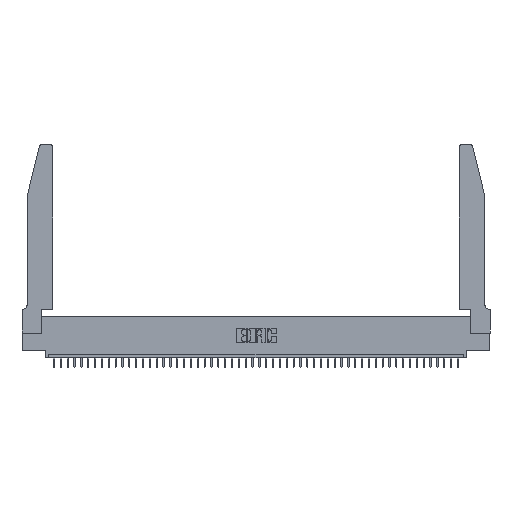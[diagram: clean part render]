
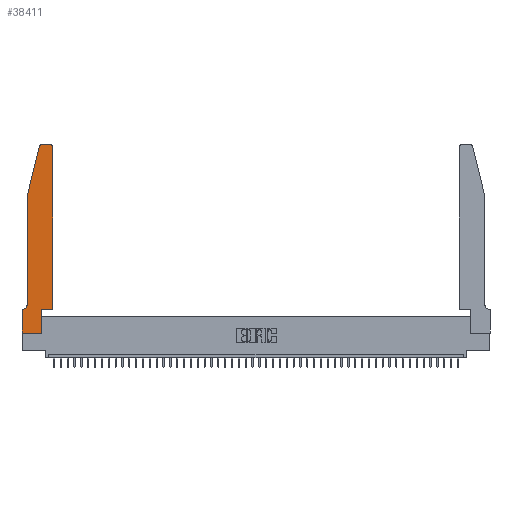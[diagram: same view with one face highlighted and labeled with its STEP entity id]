
A CAD part, top view. The second image highlights one B-rep face of the part: STEP entity #38411.
In plain terms, the highlighted planar face has unit normal (0, 0, 1).
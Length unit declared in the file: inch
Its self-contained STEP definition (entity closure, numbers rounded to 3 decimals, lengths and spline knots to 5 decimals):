
#717 = CARTESIAN_POINT ( 'NONE',  ( 0., 0., 0.37 ) ) ;
#870 = VERTEX_POINT ( 'NONE', #27815 ) ;
#1049 = VERTEX_POINT ( 'NONE', #7012 ) ;
#1482 = LINE ( 'NONE', #16204, #45130 ) ;
#1891 = LINE ( 'NONE', #32333, #27914 ) ;
#1968 = CARTESIAN_POINT ( 'NONE',  ( 0.284, 2.75, 0.37 ) ) ;
#2046 = EDGE_CURVE ( 'NONE', #19567, #12857, #1482, .T. ) ;
#2051 = ORIENTED_EDGE ( 'NONE', *, *, #29440, .T. ) ;
#2281 = VERTEX_POINT ( 'NONE', #28807 ) ;
#2352 = EDGE_CURVE ( 'NONE', #36079, #19567, #11981, .T. ) ;
#2806 = CARTESIAN_POINT ( 'NONE',  ( 0., 0., 0.37 ) ) ;
#3188 = LINE ( 'NONE', #10214, #9476 ) ;
#3370 = DIRECTION ( 'NONE',  ( 0., 0., -1. ) ) ;
#3451 = VECTOR ( 'NONE', #38414, 39.37008 ) ;
#3465 = ORIENTED_EDGE ( 'NONE', *, *, #21315, .T. ) ;
#3543 = EDGE_CURVE ( 'NONE', #21553, #870, #6575, .T. ) ;
#3619 = CARTESIAN_POINT ( 'NONE',  ( 0.284, 2.72, 0.37 ) ) ;
#3677 = VECTOR ( 'NONE', #18370, 39.37008 ) ;
#3889 = ORIENTED_EDGE ( 'NONE', *, *, #36716, .T. ) ;
#4302 = EDGE_CURVE ( 'NONE', #1049, #45081, #12167, .T. ) ;
#4757 = CARTESIAN_POINT ( 'NONE',  ( 0.2865, 0., 0.37 ) ) ;
#5993 = EDGE_CURVE ( 'NONE', #36864, #1049, #36956, .T. ) ;
#6575 = CIRCLE ( 'NONE', #32847, 0.03 ) ;
#6764 = CARTESIAN_POINT ( 'NONE',  ( 0.0055, 0.35, 0.37 ) ) ;
#7012 = CARTESIAN_POINT ( 'NONE',  ( 0.2865, 0.35, 0.37 ) ) ;
#7021 = DIRECTION ( 'NONE',  ( -1., 0., 0. ) ) ;
#7622 = CARTESIAN_POINT ( 'NONE',  ( 0.4505, 0.35, 0.37 ) ) ;
#7900 = VECTOR ( 'NONE', #8392, 39.37008 ) ;
#8392 = DIRECTION ( 'NONE',  ( -0.239, -0.971, 0. ) ) ;
#8603 = AXIS2_PLACEMENT_3D ( 'NONE', #24599, #13689, #39295 ) ;
#9476 = VECTOR ( 'NONE', #46400, 39.37008 ) ;
#10214 = CARTESIAN_POINT ( 'NONE',  ( 0.4505, 0.35, 0.37 ) ) ;
#11208 = ORIENTED_EDGE ( 'NONE', *, *, #15468, .T. ) ;
#11301 = VERTEX_POINT ( 'NONE', #24038 ) ;
#11664 = CIRCLE ( 'NONE', #8603, 0.03 ) ;
#11981 = CIRCLE ( 'NONE', #20401, 0.07 ) ;
#12167 = LINE ( 'NONE', #7622, #12753 ) ;
#12753 = VECTOR ( 'NONE', #45010, 39.37008 ) ;
#12776 = VECTOR ( 'NONE', #41845, 39.37008 ) ;
#12857 = VERTEX_POINT ( 'NONE', #22912 ) ;
#12887 = ORIENTED_EDGE ( 'NONE', *, *, #13401, .T. ) ;
#13401 = EDGE_CURVE ( 'NONE', #45081, #42775, #3188, .T. ) ;
#13453 = DIRECTION ( 'NONE',  ( 0., -1., 0. ) ) ;
#13689 = DIRECTION ( 'NONE',  ( 0., 0., 1. ) ) ;
#13905 = DIRECTION ( 'NONE',  ( 1., 0., 0. ) ) ;
#14126 = DIRECTION ( 'NONE',  ( 0., 0., 1. ) ) ;
#15296 = VERTEX_POINT ( 'NONE', #717 ) ;
#15468 = EDGE_CURVE ( 'NONE', #12857, #15296, #1891, .T. ) ;
#15611 = CARTESIAN_POINT ( 'NONE',  ( 0.0755, 2., 0.37 ) ) ;
#15855 = EDGE_CURVE ( 'NONE', #870, #11301, #37579, .T. ) ;
#16147 = CARTESIAN_POINT ( 'NONE',  ( 0.4505, 2.72, 0.37 ) ) ;
#16204 = CARTESIAN_POINT ( 'NONE',  ( 0.0755, 0.35, 0.37 ) ) ;
#16730 = VECTOR ( 'NONE', #13905, 39.37008 ) ;
#17084 = ORIENTED_EDGE ( 'NONE', *, *, #2046, .T. ) ;
#17548 = FACE_OUTER_BOUND ( 'NONE', #40872, .T. ) ;
#18370 = DIRECTION ( 'NONE',  ( 0., 1., 0. ) ) ;
#19567 = VERTEX_POINT ( 'NONE', #6764 ) ;
#20401 = AXIS2_PLACEMENT_3D ( 'NONE', #29280, #3370, #7021 ) ;
#20871 = EDGE_CURVE ( 'NONE', #11301, #36079, #23765, .T. ) ;
#21315 = EDGE_CURVE ( 'NONE', #2281, #21553, #23950, .T. ) ;
#21553 = VERTEX_POINT ( 'NONE', #1968 ) ;
#22912 = CARTESIAN_POINT ( 'NONE',  ( 0., 0.35, 0.37 ) ) ;
#23514 = CARTESIAN_POINT ( 'NONE',  ( 0.0755, 0.42, 0.37 ) ) ;
#23765 = LINE ( 'NONE', #34669, #12776 ) ;
#23950 = LINE ( 'NONE', #44954, #3451 ) ;
#24038 = CARTESIAN_POINT ( 'NONE',  ( 0.0755, 2., 0.37 ) ) ;
#24599 = CARTESIAN_POINT ( 'NONE',  ( 0.4205, 2.72, 0.37 ) ) ;
#27815 = CARTESIAN_POINT ( 'NONE',  ( 0.25487, 2.72718, 0.37 ) ) ;
#27914 = VECTOR ( 'NONE', #13453, 39.37008 ) ;
#27925 = ORIENTED_EDGE ( 'NONE', *, *, #4302, .T. ) ;
#28807 = CARTESIAN_POINT ( 'NONE',  ( 0.4205, 2.75, 0.37 ) ) ;
#29140 = ORIENTED_EDGE ( 'NONE', *, *, #2352, .T. ) ;
#29280 = CARTESIAN_POINT ( 'NONE',  ( 0.0055, 0.42, 0.37 ) ) ;
#29289 = DIRECTION ( 'NONE',  ( 1., 0., 0. ) ) ;
#29440 = EDGE_CURVE ( 'NONE', #15296, #36864, #35915, .T. ) ;
#32287 = PLANE ( 'NONE',  #39508 ) ;
#32333 = CARTESIAN_POINT ( 'NONE',  ( 0., 0., 0.37 ) ) ;
#32847 = AXIS2_PLACEMENT_3D ( 'NONE', #3619, #43939, #29289 ) ;
#34669 = CARTESIAN_POINT ( 'NONE',  ( 0.0755, 2., 0.37 ) ) ;
#35915 = LINE ( 'NONE', #2806, #16730 ) ;
#36079 = VERTEX_POINT ( 'NONE', #23514 ) ;
#36134 = DIRECTION ( 'NONE',  ( 1., 0., 0. ) ) ;
#36716 = EDGE_CURVE ( 'NONE', #42775, #2281, #11664, .T. ) ;
#36864 = VERTEX_POINT ( 'NONE', #4757 ) ;
#36956 = LINE ( 'NONE', #40786, #3677 ) ;
#37579 = LINE ( 'NONE', #15611, #7900 ) ;
#38411 = ADVANCED_FACE ( 'NONE', ( #17548 ), #32287, .T. ) ;
#38414 = DIRECTION ( 'NONE',  ( -1., 0., 0. ) ) ;
#39295 = DIRECTION ( 'NONE',  ( 1., 0., 0. ) ) ;
#39508 = AXIS2_PLACEMENT_3D ( 'NONE', #46954, #14126, #36134 ) ;
#39968 = ORIENTED_EDGE ( 'NONE', *, *, #3543, .T. ) ;
#40786 = CARTESIAN_POINT ( 'NONE',  ( 0.2865, 0.35, 0.37 ) ) ;
#40872 = EDGE_LOOP ( 'NONE', ( #3465, #39968, #41396, #45510, #29140, #17084, #11208, #2051, #45895, #27925, #12887, #3889 ) ) ;
#41396 = ORIENTED_EDGE ( 'NONE', *, *, #15855, .T. ) ;
#41845 = DIRECTION ( 'NONE',  ( 0., -1., 0. ) ) ;
#42775 = VERTEX_POINT ( 'NONE', #16147 ) ;
#42843 = CARTESIAN_POINT ( 'NONE',  ( 0.4505, 0.35, 0.37 ) ) ;
#43939 = DIRECTION ( 'NONE',  ( 0., 0., 1. ) ) ;
#44954 = CARTESIAN_POINT ( 'NONE',  ( 0.2605, 2.75, 0.37 ) ) ;
#45010 = DIRECTION ( 'NONE',  ( 1., 0., 0. ) ) ;
#45081 = VERTEX_POINT ( 'NONE', #42843 ) ;
#45130 = VECTOR ( 'NONE', #45167, 39.37008 ) ;
#45167 = DIRECTION ( 'NONE',  ( -1., 0., 0. ) ) ;
#45510 = ORIENTED_EDGE ( 'NONE', *, *, #20871, .T. ) ;
#45895 = ORIENTED_EDGE ( 'NONE', *, *, #5993, .T. ) ;
#46400 = DIRECTION ( 'NONE',  ( 0., 1., 0. ) ) ;
#46954 = CARTESIAN_POINT ( 'NONE',  ( 0., 0.35, 0.37 ) ) ;
